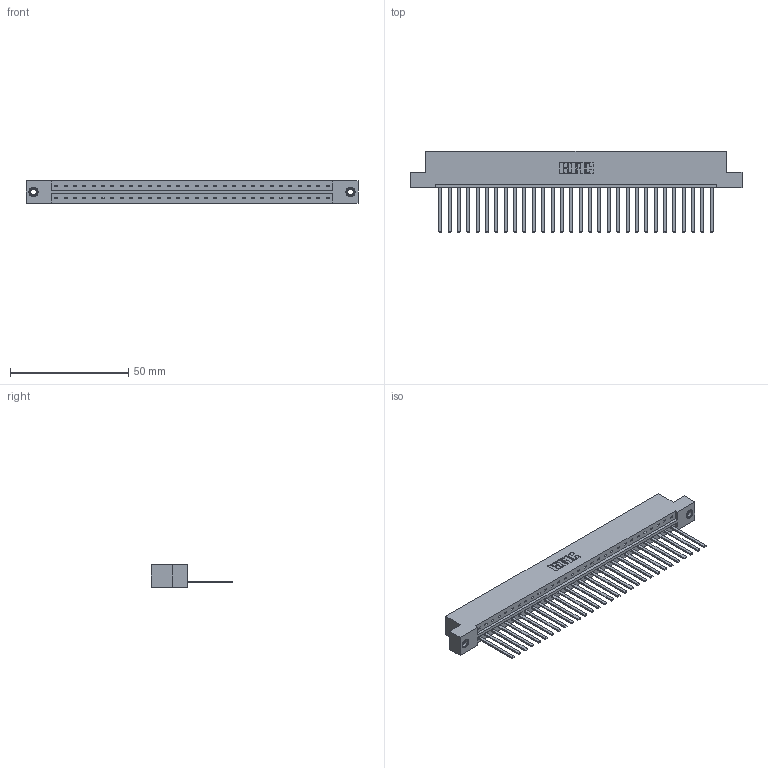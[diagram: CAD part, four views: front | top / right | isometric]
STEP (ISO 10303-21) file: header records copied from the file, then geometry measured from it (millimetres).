
FILE_DESCRIPTION (( 'STEP AP203' ), '1' );
FILE_NAME ('333-030-544-107.STEP', '2018-08-02T18:17:56', ( '' ), ( '' ), 'SwSTEP 2.0', 'SolidWorks 2016', '' );
FILE_SCHEMA (( 'CONFIG_CONTROL_DESIGN' ));
Length unit declared in the file: inch
Products named in the file (4): 345-250-001_345-250-005-103; 333-030-544-107; 345-292-001_345-293-144; 333 Part_Flush - .156 Dia - TI
Assembly tree (33 placements, depth 2):
  333-030-544-107
    333 Part_Flush - .156 Dia - TI
    345-292-001_345-293-144  x30
    345-250-001_345-250-005-103  x2
Bounding box: 140.41 x 34.3 x 9.4 mm (x, y, z)
Volume: 14360 mm3; surface area: 16626.1 mm2
Topology: 33 solids, 33 shells, 1734 faces, 5187 edges, 3410 vertices
Faces by surface type: plane 1242, cylinder 476, cone 12, torus 4
Entity records: 20894 total; most frequent: CARTESIAN_POINT 3587, ORIENTED_EDGE 3546, DIRECTION 3079, EDGE_CURVE 1773, LINE 1629, VECTOR 1629, VERTEX_POINT 1176, AXIS2_PLACEMENT_3D 725
